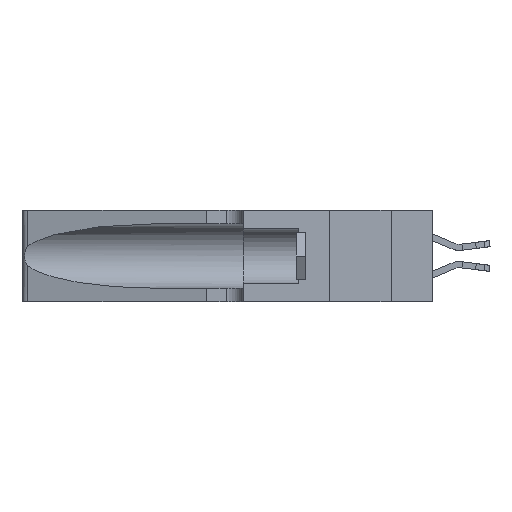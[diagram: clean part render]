
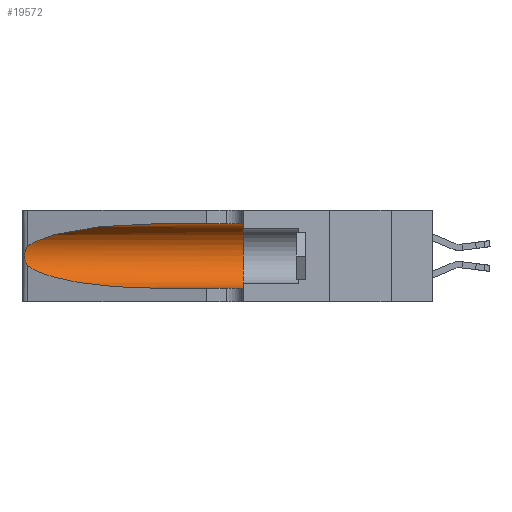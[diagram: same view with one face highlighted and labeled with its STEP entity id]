
A CAD part, left-side view. The second image highlights one B-rep face of the part: STEP entity #19572.
In plain terms, the highlighted cylindrical face has radius 3.308 mm (diameter 6.617 mm), a partial arc.
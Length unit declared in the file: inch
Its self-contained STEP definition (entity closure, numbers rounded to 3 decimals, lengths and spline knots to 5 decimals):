
#191 = CARTESIAN_POINT ( 'NONE',  ( 0.25555, 1.22994, 0.2215 ) ) ;
#927 = EDGE_LOOP ( 'NONE', ( #21453, #4563, #8082, #2770, #35258, #11409 ) ) ;
#1925 = EDGE_CURVE ( 'NONE', #18539, #35915, #35711, .T. ) ;
#2043 = DIRECTION ( 'NONE',  ( 0., 0., 1. ) ) ;
#2188 = CARTESIAN_POINT ( 'NONE',  ( 0.1305, 0.72297, 0.05475 ) ) ;
#2770 = ORIENTED_EDGE ( 'NONE', *, *, #23437, .T. ) ;
#2785 =( BOUNDED_CURVE ( )  B_SPLINE_CURVE ( 3, ( #22493, #27849, #19295, #2188 ),
 .UNSPECIFIED., .F., .T. ) 
 B_SPLINE_CURVE_WITH_KNOTS ( ( 4, 4 ),
 ( 3.44316, 4.71239 ),
 .UNSPECIFIED. ) 
 CURVE ( )  GEOMETRIC_REPRESENTATION_ITEM ( )  RATIONAL_B_SPLINE_CURVE ( ( 1., 0.87, 0.87, 1. ) ) 
 REPRESENTATION_ITEM ( '' )  );
#2918 = CARTESIAN_POINT ( 'NONE',  ( 0.18966, 0.96281, 0.31525 ) ) ;
#2930 = CARTESIAN_POINT ( 'NONE',  ( 0.26017, 1.23833, 0.17102 ) ) ;
#3055 = CARTESIAN_POINT ( 'NONE',  ( 0.25787, 1.23484, 0.2124 ) ) ;
#3287 = CARTESIAN_POINT ( 'NONE',  ( 0.25487, 1.22718, 0.14631 ) ) ;
#3676 = CARTESIAN_POINT ( 'NONE',  ( 0.1305, 1.61858, 0.31525 ) ) ;
#3945 = VECTOR ( 'NONE', #26466, 39.37008 ) ;
#4563 = ORIENTED_EDGE ( 'NONE', *, *, #34729, .T. ) ;
#4950 = VERTEX_POINT ( 'NONE', #18881 ) ;
#5200 = VERTEX_POINT ( 'NONE', #31024 ) ;
#7138 = AXIS2_PLACEMENT_3D ( 'NONE', #27118, #33325, #7924 ) ;
#7821 = B_SPLINE_CURVE_WITH_KNOTS ( 'NONE', 3,
 ( #31314, #191, #23249, #3055, #28700, #17071, #11794, #25740, #2930, #31683, #14702, #34445, #20408, #3287 ),
 .UNSPECIFIED., .F., .F.,
 ( 4, 2, 2, 2, 2, 2, 4 ),
 ( 0., 0.00027, 0.00053, 0.00107, 0.0016, 0.00187, 0.00214 ),
 .UNSPECIFIED. ) ;
#7924 = DIRECTION ( 'NONE',  ( 0., 0., -1. ) ) ;
#8082 = ORIENTED_EDGE ( 'NONE', *, *, #36570, .T. ) ;
#9954 = VECTOR ( 'NONE', #13956, 39.37008 ) ;
#10678 = CARTESIAN_POINT ( 'NONE',  ( 0.1305, 0.72297, 0.05475 ) ) ;
#11220 = CARTESIAN_POINT ( 'NONE',  ( 0.25487, 1.22718, 0.22369 ) ) ;
#11409 = ORIENTED_EDGE ( 'NONE', *, *, #16936, .F. ) ;
#11425 = CARTESIAN_POINT ( 'NONE',  ( 0.1305, 0.72297, 0.31525 ) ) ;
#11547 = LINE ( 'NONE', #3676, #3945 ) ;
#11794 = CARTESIAN_POINT ( 'NONE',  ( 0.26075, 1.23896, 0.19203 ) ) ;
#13956 = DIRECTION ( 'NONE',  ( 0., -1., 0. ) ) ;
#14435 = CARTESIAN_POINT ( 'NONE',  ( 0.2373, 1.15595, 0.28018 ) ) ;
#14702 = CARTESIAN_POINT ( 'NONE',  ( 0.25789, 1.23486, 0.15765 ) ) ;
#16075 = FACE_OUTER_BOUND ( 'NONE', #927, .T. ) ;
#16936 = EDGE_CURVE ( 'NONE', #18539, #5200, #11547, .T. ) ;
#17071 = CARTESIAN_POINT ( 'NONE',  ( 0.26018, 1.23835, 0.19895 ) ) ;
#18539 = VERTEX_POINT ( 'NONE', #25026 ) ;
#18881 = CARTESIAN_POINT ( 'NONE',  ( 0.25487, 1.22718, 0.14631 ) ) ;
#19295 = CARTESIAN_POINT ( 'NONE',  ( 0.18966, 0.96281, 0.05475 ) ) ;
#19572 = ADVANCED_FACE ( 'NONE', ( #16075 ), #26269, .F. ) ;
#20408 = CARTESIAN_POINT ( 'NONE',  ( 0.25555, 1.22993, 0.14849 ) ) ;
#21453 = ORIENTED_EDGE ( 'NONE', *, *, #1925, .T. ) ;
#22431 = LINE ( 'NONE', #32979, #9954 ) ;
#22493 = CARTESIAN_POINT ( 'NONE',  ( 0.25487, 1.22718, 0.14631 ) ) ;
#23249 = CARTESIAN_POINT ( 'NONE',  ( 0.25639, 1.23184, 0.21858 ) ) ;
#23437 = EDGE_CURVE ( 'NONE', #36567, #25470, #22431, .T. ) ;
#24852 = DIRECTION ( 'NONE',  ( 0., 1., 0. ) ) ;
#25026 = CARTESIAN_POINT ( 'NONE',  ( 0.1305, 0.72297, 0.31525 ) ) ;
#25470 = VERTEX_POINT ( 'NONE', #31056 ) ;
#25740 = CARTESIAN_POINT ( 'NONE',  ( 0.26075, 1.23896, 0.178 ) ) ;
#26269 = CYLINDRICAL_SURFACE ( 'NONE', #7138, 0.13025 ) ;
#26466 = DIRECTION ( 'NONE',  ( 0., -1., 0. ) ) ;
#27118 = CARTESIAN_POINT ( 'NONE',  ( 0.1305, 1.61858, 0.185 ) ) ;
#27849 = CARTESIAN_POINT ( 'NONE',  ( 0.2373, 1.15595, 0.08982 ) ) ;
#28700 = CARTESIAN_POINT ( 'NONE',  ( 0.25854, 1.2359, 0.20912 ) ) ;
#28717 = CIRCLE ( 'NONE', #34988, 0.13025 ) ;
#28756 = EDGE_CURVE ( 'NONE', #5200, #25470, #28717, .T. ) ;
#30441 = CARTESIAN_POINT ( 'NONE',  ( 0.1305, 0.35, 0.185 ) ) ;
#31024 = CARTESIAN_POINT ( 'NONE',  ( 0.1305, 0.35, 0.31525 ) ) ;
#31056 = CARTESIAN_POINT ( 'NONE',  ( 0.1305, 0.35, 0.05475 ) ) ;
#31314 = CARTESIAN_POINT ( 'NONE',  ( 0.25487, 1.22718, 0.22369 ) ) ;
#31683 = CARTESIAN_POINT ( 'NONE',  ( 0.25856, 1.23593, 0.16098 ) ) ;
#32979 = CARTESIAN_POINT ( 'NONE',  ( 0.1305, 1.61858, 0.05475 ) ) ;
#33325 = DIRECTION ( 'NONE',  ( 0., -1., 0. ) ) ;
#34316 = CARTESIAN_POINT ( 'NONE',  ( 0.25487, 1.22718, 0.22369 ) ) ;
#34445 = CARTESIAN_POINT ( 'NONE',  ( 0.25639, 1.23186, 0.15144 ) ) ;
#34729 = EDGE_CURVE ( 'NONE', #35915, #4950, #7821, .T. ) ;
#34988 = AXIS2_PLACEMENT_3D ( 'NONE', #30441, #24852, #2043 ) ;
#35258 = ORIENTED_EDGE ( 'NONE', *, *, #28756, .F. ) ;
#35711 =( BOUNDED_CURVE ( )  B_SPLINE_CURVE ( 3, ( #11425, #2918, #14435, #34316 ),
 .UNSPECIFIED., .F., .T. ) 
 B_SPLINE_CURVE_WITH_KNOTS ( ( 4, 4 ),
 ( 1.5708, 2.84003 ),
 .UNSPECIFIED. ) 
 CURVE ( )  GEOMETRIC_REPRESENTATION_ITEM ( )  RATIONAL_B_SPLINE_CURVE ( ( 1., 0.87, 0.87, 1. ) ) 
 REPRESENTATION_ITEM ( '' )  );
#35915 = VERTEX_POINT ( 'NONE', #11220 ) ;
#36567 = VERTEX_POINT ( 'NONE', #10678 ) ;
#36570 = EDGE_CURVE ( 'NONE', #4950, #36567, #2785, .T. ) ;
